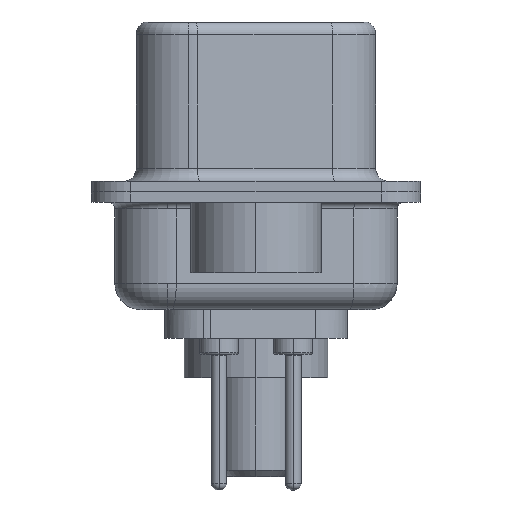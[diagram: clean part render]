
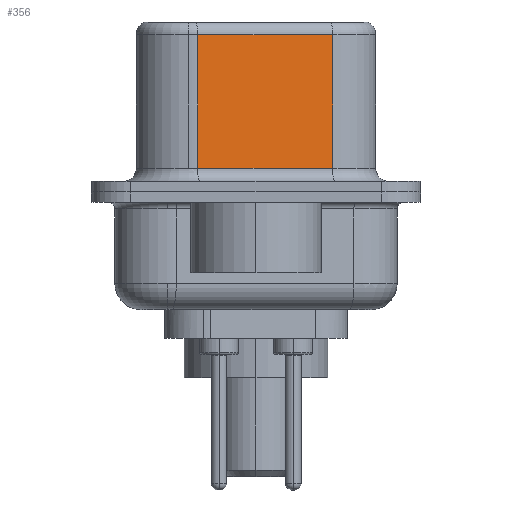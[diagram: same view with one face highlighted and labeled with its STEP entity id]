
A CAD part, left-side view. The second image highlights one B-rep face of the part: STEP entity #356.
In plain terms, the highlighted planar face has unit normal (-0.985, -0.174, 0).
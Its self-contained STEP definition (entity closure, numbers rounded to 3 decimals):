
#303 = EDGE_CURVE ( 'NONE', #11136, #6474, #7239, .T. ) ;
#356 = ADVANCED_FACE ( 'NONE', ( #2994 ), #13442, .F. ) ;
#812 = CARTESIAN_POINT ( 'NONE',  ( 4.565, -2.927, 6.02 ) ) ;
#871 = DIRECTION ( 'NONE',  ( 0.985, 0.174, 0. ) ) ;
#1268 = VECTOR ( 'NONE', #9933, 1000. ) ;
#1390 = DIRECTION ( 'NONE',  ( 0.174, -0.985, 0. ) ) ;
#1472 = LINE ( 'NONE', #6984, #7987 ) ;
#1983 = VECTOR ( 'NONE', #13291, 1000. ) ;
#2944 = EDGE_CURVE ( 'NONE', #10418, #6474, #1472, .T. ) ;
#2994 = FACE_OUTER_BOUND ( 'NONE', #16255, .T. ) ;
#3876 = CARTESIAN_POINT ( 'NONE',  ( 3.655, 2.233, 6.02 ) ) ;
#3948 = CARTESIAN_POINT ( 'NONE',  ( 4.565, -2.927, 6.02 ) ) ;
#3969 = ORIENTED_EDGE ( 'NONE', *, *, #9922, .T. ) ;
#4098 = CARTESIAN_POINT ( 'NONE',  ( 3.655, 2.233, 6.52 ) ) ;
#4749 = LINE ( 'NONE', #812, #1268 ) ;
#5039 = LINE ( 'NONE', #4098, #1983 ) ;
#5052 = CARTESIAN_POINT ( 'NONE',  ( 3.655, 2.233, 0.9 ) ) ;
#6474 = VERTEX_POINT ( 'NONE', #6860 ) ;
#6761 = CARTESIAN_POINT ( 'NONE',  ( 4.565, -2.927, 6.52 ) ) ;
#6860 = CARTESIAN_POINT ( 'NONE',  ( 4.565, -2.927, 0.9 ) ) ;
#6984 = CARTESIAN_POINT ( 'NONE',  ( 4.565, -2.927, 0.9 ) ) ;
#7239 = LINE ( 'NONE', #14186, #10755 ) ;
#7410 = ORIENTED_EDGE ( 'NONE', *, *, #2944, .T. ) ;
#7987 = VECTOR ( 'NONE', #1390, 1000. ) ;
#8867 = DIRECTION ( 'NONE',  ( 0., 0., -1. ) ) ;
#9349 = AXIS2_PLACEMENT_3D ( 'NONE', #6761, #871, #11907 ) ;
#9826 = VERTEX_POINT ( 'NONE', #3876 ) ;
#9922 = EDGE_CURVE ( 'NONE', #9826, #10418, #5039, .T. ) ;
#9933 = DIRECTION ( 'NONE',  ( -0.174, 0.985, 0. ) ) ;
#10092 = ORIENTED_EDGE ( 'NONE', *, *, #303, .F. ) ;
#10418 = VERTEX_POINT ( 'NONE', #5052 ) ;
#10755 = VECTOR ( 'NONE', #8867, 1000. ) ;
#11136 = VERTEX_POINT ( 'NONE', #3948 ) ;
#11907 = DIRECTION ( 'NONE',  ( -0.174, 0.985, 0. ) ) ;
#13080 = EDGE_CURVE ( 'NONE', #11136, #9826, #4749, .T. ) ;
#13291 = DIRECTION ( 'NONE',  ( 0., 0., -1. ) ) ;
#13442 = PLANE ( 'NONE',  #9349 ) ;
#13635 = ORIENTED_EDGE ( 'NONE', *, *, #13080, .T. ) ;
#14186 = CARTESIAN_POINT ( 'NONE',  ( 4.565, -2.927, 6.52 ) ) ;
#16255 = EDGE_LOOP ( 'NONE', ( #10092, #13635, #3969, #7410 ) ) ;
